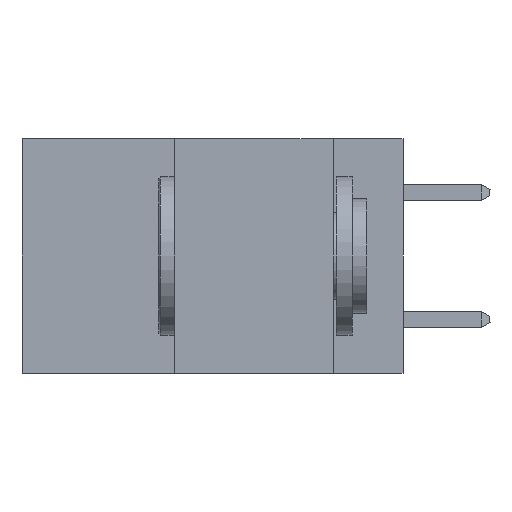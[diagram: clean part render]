
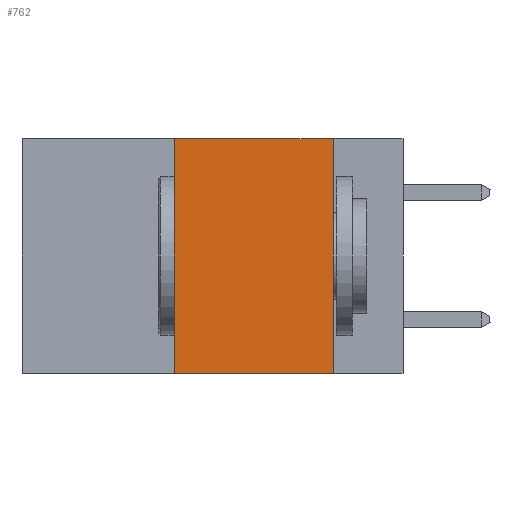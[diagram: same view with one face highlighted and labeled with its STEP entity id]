
A CAD part, left-side view. The second image highlights one B-rep face of the part: STEP entity #762.
In plain terms, the highlighted planar face has unit normal (-1, 0, 0).
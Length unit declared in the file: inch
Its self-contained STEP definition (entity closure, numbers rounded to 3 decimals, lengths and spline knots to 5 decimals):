
#762 = ADVANCED_FACE ( 'NONE', ( #2876 ), #18551, .F. ) ;
#1666 = EDGE_CURVE ( 'NONE', #24123, #20597, #3780, .T. ) ;
#2876 = FACE_OUTER_BOUND ( 'NONE', #17704, .T. ) ;
#3620 = AXIS2_PLACEMENT_3D ( 'NONE', #4599, #18160, #31914 ) ;
#3780 = LINE ( 'NONE', #21147, #9361 ) ;
#3877 = DIRECTION ( 'NONE',  ( 0., 0., 1. ) ) ;
#4599 = CARTESIAN_POINT ( 'NONE',  ( 0., 0.6, 0. ) ) ;
#5389 = VECTOR ( 'NONE', #30171, 39.37008 ) ;
#5472 = DIRECTION ( 'NONE',  ( 0., 0., -1. ) ) ;
#5578 = LINE ( 'NONE', #37733, #11589 ) ;
#9361 = VECTOR ( 'NONE', #9695, 39.37008 ) ;
#9614 = EDGE_CURVE ( 'NONE', #19126, #20563, #33955, .T. ) ;
#9641 = ORIENTED_EDGE ( 'NONE', *, *, #29884, .F. ) ;
#9695 = DIRECTION ( 'NONE',  ( 0., -1., 0. ) ) ;
#10445 = ORIENTED_EDGE ( 'NONE', *, *, #1666, .T. ) ;
#11589 = VECTOR ( 'NONE', #5472, 39.37008 ) ;
#12086 = ORIENTED_EDGE ( 'NONE', *, *, #25702, .F. ) ;
#14127 = CARTESIAN_POINT ( 'NONE',  ( 0., 0.6, 0. ) ) ;
#16841 = LINE ( 'NONE', #23122, #29603 ) ;
#17233 = CARTESIAN_POINT ( 'NONE',  ( 0., 0.36, -0.37 ) ) ;
#17704 = EDGE_LOOP ( 'NONE', ( #9641, #18356, #12086, #10445 ) ) ;
#18160 = DIRECTION ( 'NONE',  ( 1., 0., 0. ) ) ;
#18356 = ORIENTED_EDGE ( 'NONE', *, *, #9614, .F. ) ;
#18551 = PLANE ( 'NONE',  #3620 ) ;
#18627 = CARTESIAN_POINT ( 'NONE',  ( 0., 0.11, 0. ) ) ;
#19126 = VERTEX_POINT ( 'NONE', #37594 ) ;
#20563 = VERTEX_POINT ( 'NONE', #18627 ) ;
#20597 = VERTEX_POINT ( 'NONE', #41154 ) ;
#21147 = CARTESIAN_POINT ( 'NONE',  ( 0., 0.6, -0.37 ) ) ;
#23122 = CARTESIAN_POINT ( 'NONE',  ( 0., 0.36, 0. ) ) ;
#24123 = VERTEX_POINT ( 'NONE', #17233 ) ;
#25702 = EDGE_CURVE ( 'NONE', #24123, #19126, #16841, .T. ) ;
#29603 = VECTOR ( 'NONE', #3877, 39.37008 ) ;
#29884 = EDGE_CURVE ( 'NONE', #20563, #20597, #5578, .T. ) ;
#30171 = DIRECTION ( 'NONE',  ( 0., -1., 0. ) ) ;
#31914 = DIRECTION ( 'NONE',  ( 0., 0., -1. ) ) ;
#33955 = LINE ( 'NONE', #14127, #5389 ) ;
#37594 = CARTESIAN_POINT ( 'NONE',  ( 0., 0.36, 0. ) ) ;
#37733 = CARTESIAN_POINT ( 'NONE',  ( 0., 0.11, 0. ) ) ;
#41154 = CARTESIAN_POINT ( 'NONE',  ( 0., 0.11, -0.37 ) ) ;
